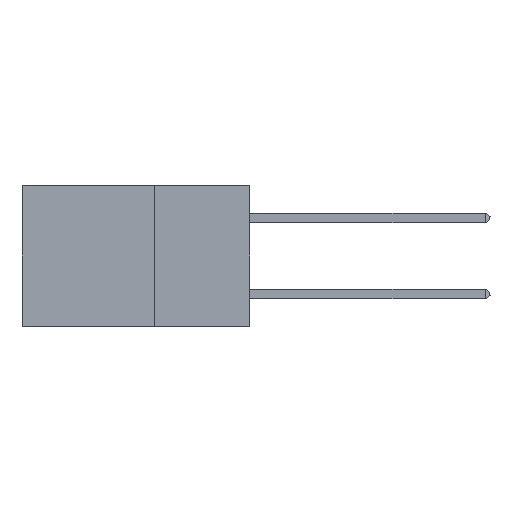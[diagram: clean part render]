
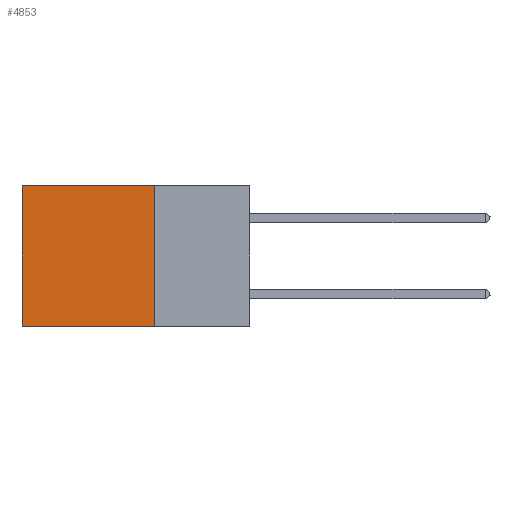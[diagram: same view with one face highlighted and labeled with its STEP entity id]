
A CAD part, left-side view. The second image highlights one B-rep face of the part: STEP entity #4853.
In plain terms, the highlighted planar face has unit normal (-1, 0, 0).
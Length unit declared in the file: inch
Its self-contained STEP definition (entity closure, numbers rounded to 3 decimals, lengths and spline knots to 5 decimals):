
#973 = DIRECTION ( 'NONE',  ( 0., 0., -1. ) ) ;
#1795 = ORIENTED_EDGE ( 'NONE', *, *, #18197, .F. ) ;
#3067 = DIRECTION ( 'NONE',  ( 0., 1., 0. ) ) ;
#4853 = ADVANCED_FACE ( 'NONE', ( #27308 ), #18372, .F. ) ;
#5978 = CARTESIAN_POINT ( 'NONE',  ( 0.2875, 0.25, 0. ) ) ;
#6496 = ORIENTED_EDGE ( 'NONE', *, *, #29736, .F. ) ;
#10844 = CARTESIAN_POINT ( 'NONE',  ( 0.2875, 0.25, 0. ) ) ;
#13812 = VECTOR ( 'NONE', #32585, 39.37008 ) ;
#14825 = CARTESIAN_POINT ( 'NONE',  ( 0.2875, 0.6, -0.37 ) ) ;
#16748 = EDGE_CURVE ( 'NONE', #17705, #31553, #32963, .T. ) ;
#17136 = LINE ( 'NONE', #32208, #29051 ) ;
#17705 = VERTEX_POINT ( 'NONE', #31434 ) ;
#17795 = CARTESIAN_POINT ( 'NONE',  ( 0.2875, 0.25, -0.37 ) ) ;
#18197 = EDGE_CURVE ( 'NONE', #17705, #22116, #28868, .T. ) ;
#18372 = PLANE ( 'NONE',  #21768 ) ;
#21768 = AXIS2_PLACEMENT_3D ( 'NONE', #5978, #23847, #973 ) ;
#22116 = VERTEX_POINT ( 'NONE', #23890 ) ;
#23288 = CARTESIAN_POINT ( 'NONE',  ( 0.2875, 0.25, 0. ) ) ;
#23739 = VERTEX_POINT ( 'NONE', #14825 ) ;
#23847 = DIRECTION ( 'NONE',  ( 1., 0., 0. ) ) ;
#23890 = CARTESIAN_POINT ( 'NONE',  ( 0.2875, 0.25, -0.37 ) ) ;
#24447 = ORIENTED_EDGE ( 'NONE', *, *, #16748, .T. ) ;
#24816 = EDGE_LOOP ( 'NONE', ( #26051, #6496, #1795, #24447 ) ) ;
#26051 = ORIENTED_EDGE ( 'NONE', *, *, #27059, .T. ) ;
#26150 = CARTESIAN_POINT ( 'NONE',  ( 0.2875, 0.6, 0. ) ) ;
#26226 = VECTOR ( 'NONE', #3067, 39.37008 ) ;
#27059 = EDGE_CURVE ( 'NONE', #31553, #23739, #17136, .T. ) ;
#27308 = FACE_OUTER_BOUND ( 'NONE', #24816, .T. ) ;
#28459 = VECTOR ( 'NONE', #28517, 39.37008 ) ;
#28507 = LINE ( 'NONE', #17795, #13812 ) ;
#28517 = DIRECTION ( 'NONE',  ( 0., 0., -1. ) ) ;
#28868 = LINE ( 'NONE', #10844, #28459 ) ;
#29051 = VECTOR ( 'NONE', #32655, 39.37008 ) ;
#29736 = EDGE_CURVE ( 'NONE', #22116, #23739, #28507, .T. ) ;
#31434 = CARTESIAN_POINT ( 'NONE',  ( 0.2875, 0.25, 0. ) ) ;
#31553 = VERTEX_POINT ( 'NONE', #26150 ) ;
#32208 = CARTESIAN_POINT ( 'NONE',  ( 0.2875, 0.6, 0. ) ) ;
#32585 = DIRECTION ( 'NONE',  ( 0., 1., 0. ) ) ;
#32655 = DIRECTION ( 'NONE',  ( 0., 0., -1. ) ) ;
#32963 = LINE ( 'NONE', #23288, #26226 ) ;
